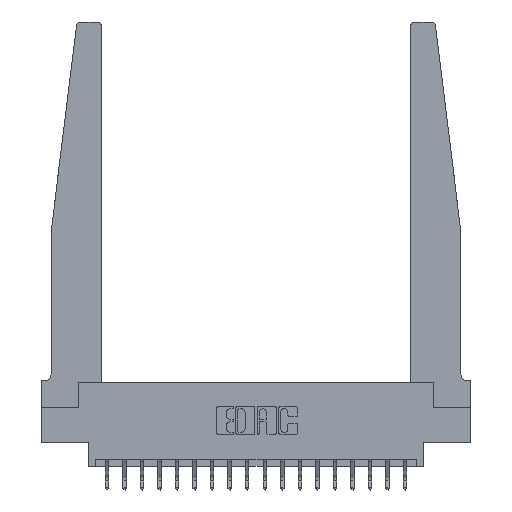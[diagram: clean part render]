
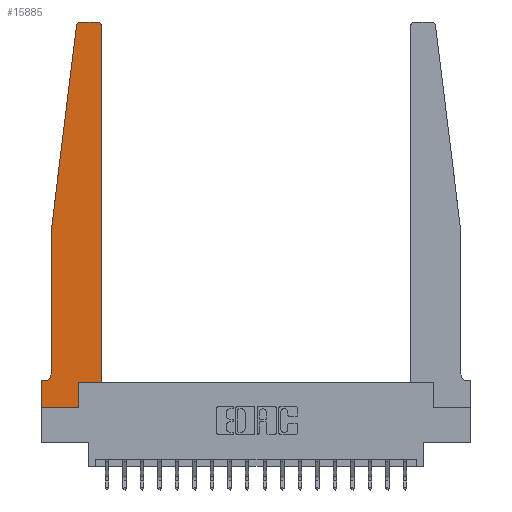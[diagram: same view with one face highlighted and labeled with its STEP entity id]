
A CAD part, top view. The second image highlights one B-rep face of the part: STEP entity #15885.
In plain terms, the highlighted planar face has unit normal (0, 0, 1).
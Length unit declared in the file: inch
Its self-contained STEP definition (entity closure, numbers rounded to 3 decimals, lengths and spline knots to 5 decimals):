
#45 = EDGE_CURVE ( 'NONE', #8764, #3204, #1997, .T. ) ;
#60 = LINE ( 'NONE', #18794, #19612 ) ;
#153 = CARTESIAN_POINT ( 'NONE',  ( 0.24675, 2.72367, 0.37 ) ) ;
#183 = EDGE_CURVE ( 'NONE', #17963, #3274, #12784, .T. ) ;
#384 = DIRECTION ( 'NONE',  ( -0.122, -0.992, 0. ) ) ;
#749 = VERTEX_POINT ( 'NONE', #5503 ) ;
#865 = CARTESIAN_POINT ( 'NONE',  ( 0.015, 0.2375, 0.37 ) ) ;
#1192 = EDGE_LOOP ( 'NONE', ( #5077, #11918, #2707, #7078, #8895, #15906, #7672, #11736, #16954, #9570, #8946, #20223 ) ) ;
#1398 = AXIS2_PLACEMENT_3D ( 'NONE', #865, #15301, #18228 ) ;
#1413 = EDGE_CURVE ( 'NONE', #14759, #18534, #10778, .T. ) ;
#1478 = DIRECTION ( 'NONE',  ( 0., 0., 1. ) ) ;
#1664 = DIRECTION ( 'NONE',  ( 1., 0., 0. ) ) ;
#1997 = CIRCLE ( 'NONE', #5292, 0.03 ) ;
#2266 = DIRECTION ( 'NONE',  ( 1., 0., 0. ) ) ;
#2388 = CARTESIAN_POINT ( 'NONE',  ( 0.27653, 2.75, 0.37 ) ) ;
#2434 = EDGE_CURVE ( 'NONE', #16052, #5039, #11092, .T. ) ;
#2547 = VECTOR ( 'NONE', #384, 39.37008 ) ;
#2707 = ORIENTED_EDGE ( 'NONE', *, *, #16418, .T. ) ;
#2726 = CARTESIAN_POINT ( 'NONE',  ( 0., 0., 0.37 ) ) ;
#2930 = LINE ( 'NONE', #2726, #6270 ) ;
#2978 = CARTESIAN_POINT ( 'NONE',  ( 0., 0.1875, 0.37 ) ) ;
#3204 = VERTEX_POINT ( 'NONE', #18556 ) ;
#3274 = VERTEX_POINT ( 'NONE', #2978 ) ;
#5039 = VERTEX_POINT ( 'NONE', #18853 ) ;
#5077 = ORIENTED_EDGE ( 'NONE', *, *, #10680, .T. ) ;
#5292 = AXIS2_PLACEMENT_3D ( 'NONE', #11025, #12635, #1664 ) ;
#5503 = CARTESIAN_POINT ( 'NONE',  ( 0., 0., 0.37 ) ) ;
#6065 = VECTOR ( 'NONE', #15546, 39.37008 ) ;
#6270 = VECTOR ( 'NONE', #12371, 39.37008 ) ;
#6315 = DIRECTION ( 'NONE',  ( 1., 0., 0. ) ) ;
#6495 = CIRCLE ( 'NONE', #18156, 0.03 ) ;
#6636 = VECTOR ( 'NONE', #17718, 39.37008 ) ;
#6904 = CARTESIAN_POINT ( 'NONE',  ( 0., 0., 0.37 ) ) ;
#7042 = LINE ( 'NONE', #10268, #2547 ) ;
#7078 = ORIENTED_EDGE ( 'NONE', *, *, #2434, .T. ) ;
#7096 = EDGE_CURVE ( 'NONE', #5039, #17963, #13938, .T. ) ;
#7418 = VECTOR ( 'NONE', #9209, 39.37008 ) ;
#7672 = ORIENTED_EDGE ( 'NONE', *, *, #8086, .T. ) ;
#7898 = FACE_OUTER_BOUND ( 'NONE', #1192, .T. ) ;
#8086 = EDGE_CURVE ( 'NONE', #3274, #749, #13039, .T. ) ;
#8433 = DIRECTION ( 'NONE',  ( -1., 0., 0. ) ) ;
#8707 = CARTESIAN_POINT ( 'NONE',  ( 0.27653, 2.72, 0.37 ) ) ;
#8712 = CARTESIAN_POINT ( 'NONE',  ( 0.425, 0.18, 0.37 ) ) ;
#8764 = VERTEX_POINT ( 'NONE', #15840 ) ;
#8895 = ORIENTED_EDGE ( 'NONE', *, *, #7096, .T. ) ;
#8946 = ORIENTED_EDGE ( 'NONE', *, *, #15369, .T. ) ;
#9206 = CARTESIAN_POINT ( 'NONE',  ( 0.2605, 0.18, 0.37 ) ) ;
#9207 = CARTESIAN_POINT ( 'NONE',  ( 0.425, 0.18, 0.37 ) ) ;
#9209 = DIRECTION ( 'NONE',  ( 0., -1., 0. ) ) ;
#9570 = ORIENTED_EDGE ( 'NONE', *, *, #9625, .T. ) ;
#9625 = EDGE_CURVE ( 'NONE', #18534, #18106, #60, .T. ) ;
#9999 = CARTESIAN_POINT ( 'NONE',  ( 0.25, 2.75, 0.37 ) ) ;
#10268 = CARTESIAN_POINT ( 'NONE',  ( 0.065, 1.25, 0.37 ) ) ;
#10680 = EDGE_CURVE ( 'NONE', #3204, #10953, #18008, .T. ) ;
#10778 = LINE ( 'NONE', #9206, #6065 ) ;
#10953 = VERTEX_POINT ( 'NONE', #2388 ) ;
#11025 = CARTESIAN_POINT ( 'NONE',  ( 0.395, 2.72, 0.37 ) ) ;
#11092 = LINE ( 'NONE', #17423, #7418 ) ;
#11379 = CARTESIAN_POINT ( 'NONE',  ( 0.065, 0.1875, 0.37 ) ) ;
#11396 = VECTOR ( 'NONE', #8433, 39.37008 ) ;
#11736 = ORIENTED_EDGE ( 'NONE', *, *, #20314, .T. ) ;
#11918 = ORIENTED_EDGE ( 'NONE', *, *, #17132, .T. ) ;
#12121 = VECTOR ( 'NONE', #15335, 39.37008 ) ;
#12371 = DIRECTION ( 'NONE',  ( 1., 0., 0. ) ) ;
#12469 = CARTESIAN_POINT ( 'NONE',  ( 0.015, 0.1875, 0.37 ) ) ;
#12635 = DIRECTION ( 'NONE',  ( 0., 0., 1. ) ) ;
#12642 = PLANE ( 'NONE',  #14107 ) ;
#12784 = LINE ( 'NONE', #11379, #6636 ) ;
#13039 = LINE ( 'NONE', #6904, #14950 ) ;
#13478 = VERTEX_POINT ( 'NONE', #153 ) ;
#13938 = CIRCLE ( 'NONE', #1398, 0.05 ) ;
#13967 = DIRECTION ( 'NONE',  ( 1., 0., 0. ) ) ;
#14107 = AXIS2_PLACEMENT_3D ( 'NONE', #18900, #1478, #6315 ) ;
#14759 = VERTEX_POINT ( 'NONE', #15967 ) ;
#14950 = VECTOR ( 'NONE', #17643, 39.37008 ) ;
#15301 = DIRECTION ( 'NONE',  ( 0., 0., -1. ) ) ;
#15335 = DIRECTION ( 'NONE',  ( 0., 1., 0. ) ) ;
#15369 = EDGE_CURVE ( 'NONE', #18106, #8764, #17108, .T. ) ;
#15546 = DIRECTION ( 'NONE',  ( 0., 1., 0. ) ) ;
#15604 = CARTESIAN_POINT ( 'NONE',  ( 0.2605, 0.18, 0.37 ) ) ;
#15840 = CARTESIAN_POINT ( 'NONE',  ( 0.425, 2.72, 0.37 ) ) ;
#15885 = ADVANCED_FACE ( 'NONE', ( #7898 ), #12642, .T. ) ;
#15906 = ORIENTED_EDGE ( 'NONE', *, *, #183, .T. ) ;
#15967 = CARTESIAN_POINT ( 'NONE',  ( 0.2605, 0., 0.37 ) ) ;
#16052 = VERTEX_POINT ( 'NONE', #18388 ) ;
#16418 = EDGE_CURVE ( 'NONE', #13478, #16052, #7042, .T. ) ;
#16954 = ORIENTED_EDGE ( 'NONE', *, *, #1413, .T. ) ;
#17108 = LINE ( 'NONE', #9207, #12121 ) ;
#17132 = EDGE_CURVE ( 'NONE', #10953, #13478, #6495, .T. ) ;
#17423 = CARTESIAN_POINT ( 'NONE',  ( 0.065, 1.25, 0.37 ) ) ;
#17643 = DIRECTION ( 'NONE',  ( 0., -1., 0. ) ) ;
#17718 = DIRECTION ( 'NONE',  ( -1., 0., 0. ) ) ;
#17963 = VERTEX_POINT ( 'NONE', #12469 ) ;
#18008 = LINE ( 'NONE', #9999, #11396 ) ;
#18106 = VERTEX_POINT ( 'NONE', #8712 ) ;
#18156 = AXIS2_PLACEMENT_3D ( 'NONE', #8707, #18276, #13967 ) ;
#18228 = DIRECTION ( 'NONE',  ( -1., 0., 0. ) ) ;
#18276 = DIRECTION ( 'NONE',  ( 0., 0., 1. ) ) ;
#18388 = CARTESIAN_POINT ( 'NONE',  ( 0.065, 1.25, 0.37 ) ) ;
#18534 = VERTEX_POINT ( 'NONE', #15604 ) ;
#18556 = CARTESIAN_POINT ( 'NONE',  ( 0.395, 2.75, 0.37 ) ) ;
#18794 = CARTESIAN_POINT ( 'NONE',  ( 0.425, 0.18, 0.37 ) ) ;
#18853 = CARTESIAN_POINT ( 'NONE',  ( 0.065, 0.2375, 0.37 ) ) ;
#18900 = CARTESIAN_POINT ( 'NONE',  ( 0., 0.1875, 0.37 ) ) ;
#19612 = VECTOR ( 'NONE', #2266, 39.37008 ) ;
#20223 = ORIENTED_EDGE ( 'NONE', *, *, #45, .T. ) ;
#20314 = EDGE_CURVE ( 'NONE', #749, #14759, #2930, .T. ) ;
